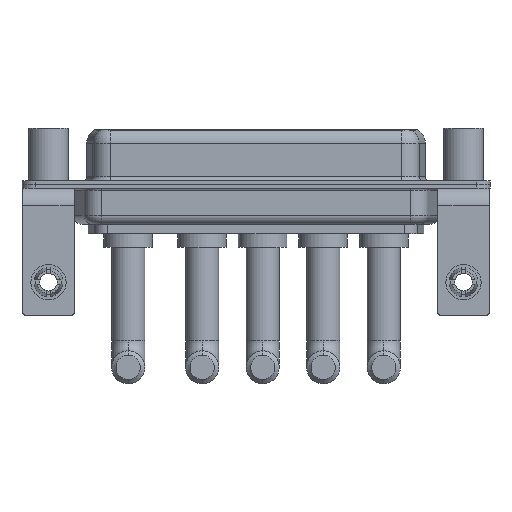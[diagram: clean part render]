
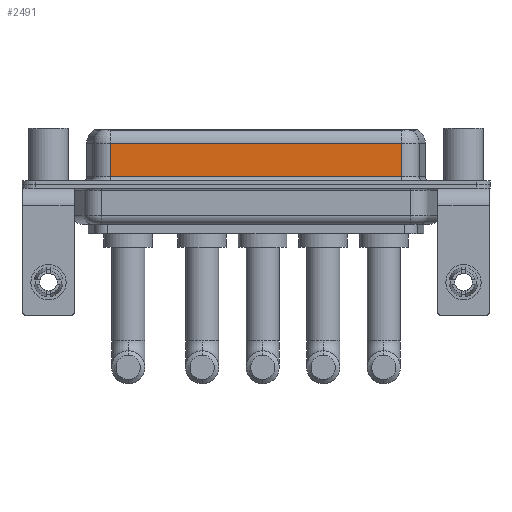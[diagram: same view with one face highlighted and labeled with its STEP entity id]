
A CAD part, front view. The second image highlights one B-rep face of the part: STEP entity #2491.
In plain terms, the highlighted planar face has unit normal (0, -1, 0).
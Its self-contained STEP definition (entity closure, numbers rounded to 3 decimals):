
#497 = ORIENTED_EDGE ( 'NONE', *, *, #12401, .T. ) ;
#917 = PLANE ( 'NONE',  #2815 ) ;
#1949 = CARTESIAN_POINT ( 'NONE',  ( 40.037, -3.95, 6.4 ) ) ;
#2444 = CARTESIAN_POINT ( 'NONE',  ( 40.037, -3.95, 6.4 ) ) ;
#2491 = ADVANCED_FACE ( 'NONE', ( #8425 ), #917, .F. ) ;
#2815 = AXIS2_PLACEMENT_3D ( 'NONE', #1949, #12278, #12521 ) ;
#3112 = VERTEX_POINT ( 'NONE', #6093 ) ;
#3543 = CARTESIAN_POINT ( 'NONE',  ( 40.037, -3.95, 4.65 ) ) ;
#3643 = LINE ( 'NONE', #2444, #10662 ) ;
#4829 = CARTESIAN_POINT ( 'NONE',  ( 40.037, -3.95, 0.9 ) ) ;
#6093 = CARTESIAN_POINT ( 'NONE',  ( 7.013, -3.95, 0.9 ) ) ;
#6118 = LINE ( 'NONE', #4829, #16531 ) ;
#6206 = DIRECTION ( 'NONE',  ( 0., 0., -1. ) ) ;
#6711 = ORIENTED_EDGE ( 'NONE', *, *, #10968, .F. ) ;
#7305 = DIRECTION ( 'NONE',  ( 1., 0., 0. ) ) ;
#7685 = ORIENTED_EDGE ( 'NONE', *, *, #7867, .T. ) ;
#7690 = LINE ( 'NONE', #10449, #13929 ) ;
#7867 = EDGE_CURVE ( 'NONE', #3112, #14441, #6118, .T. ) ;
#8301 = CARTESIAN_POINT ( 'NONE',  ( 7.013, -3.95, 4.65 ) ) ;
#8425 = FACE_OUTER_BOUND ( 'NONE', #11260, .T. ) ;
#9588 = VECTOR ( 'NONE', #12489, 1000. ) ;
#9790 = CARTESIAN_POINT ( 'NONE',  ( 40.037, -3.95, 0.9 ) ) ;
#10449 = CARTESIAN_POINT ( 'NONE',  ( 7.013, -3.95, 6.4 ) ) ;
#10662 = VECTOR ( 'NONE', #6206, 1000. ) ;
#10968 = EDGE_CURVE ( 'NONE', #14634, #14441, #3643, .T. ) ;
#11234 = LINE ( 'NONE', #3543, #9588 ) ;
#11260 = EDGE_LOOP ( 'NONE', ( #6711, #13048, #497, #7685 ) ) ;
#11651 = CARTESIAN_POINT ( 'NONE',  ( 40.037, -3.95, 4.65 ) ) ;
#12278 = DIRECTION ( 'NONE',  ( 0., 1., 0. ) ) ;
#12401 = EDGE_CURVE ( 'NONE', #16379, #3112, #7690, .T. ) ;
#12489 = DIRECTION ( 'NONE',  ( -1., 0., 0. ) ) ;
#12521 = DIRECTION ( 'NONE',  ( 0., 0., 1. ) ) ;
#12823 = DIRECTION ( 'NONE',  ( 0., 0., -1. ) ) ;
#13048 = ORIENTED_EDGE ( 'NONE', *, *, #13710, .T. ) ;
#13710 = EDGE_CURVE ( 'NONE', #14634, #16379, #11234, .T. ) ;
#13929 = VECTOR ( 'NONE', #12823, 1000. ) ;
#14441 = VERTEX_POINT ( 'NONE', #9790 ) ;
#14634 = VERTEX_POINT ( 'NONE', #11651 ) ;
#16379 = VERTEX_POINT ( 'NONE', #8301 ) ;
#16531 = VECTOR ( 'NONE', #7305, 1000. ) ;
